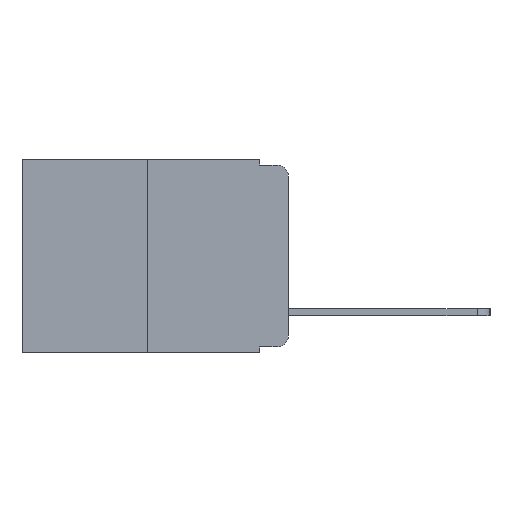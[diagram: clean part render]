
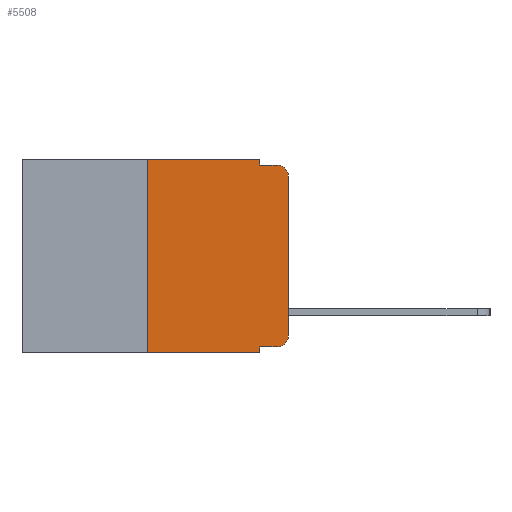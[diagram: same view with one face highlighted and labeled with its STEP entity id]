
A CAD part, left-side view. The second image highlights one B-rep face of the part: STEP entity #5508.
In plain terms, the highlighted planar face has unit normal (-1, 0, 0).
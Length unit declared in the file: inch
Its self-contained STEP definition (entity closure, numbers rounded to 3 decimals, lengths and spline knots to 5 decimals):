
#80 = VECTOR ( 'NONE', #3309, 39.37008 ) ;
#311 = VERTEX_POINT ( 'NONE', #6565 ) ;
#457 = LINE ( 'NONE', #17098, #10699 ) ;
#534 = EDGE_CURVE ( 'NONE', #11161, #9742, #10395, .T. ) ;
#926 = VERTEX_POINT ( 'NONE', #11700 ) ;
#956 = CARTESIAN_POINT ( 'NONE',  ( 0., 0.051, -0.01 ) ) ;
#980 = LINE ( 'NONE', #11636, #11213 ) ;
#1496 = CARTESIAN_POINT ( 'NONE',  ( 0., 0.051, -0.333 ) ) ;
#1633 = ORIENTED_EDGE ( 'NONE', *, *, #11664, .F. ) ;
#1896 = CARTESIAN_POINT ( 'NONE',  ( 0., 0.473, 0. ) ) ;
#2559 = LINE ( 'NONE', #1496, #16178 ) ;
#2613 = ORIENTED_EDGE ( 'NONE', *, *, #13115, .T. ) ;
#3051 = VERTEX_POINT ( 'NONE', #16866 ) ;
#3148 = ORIENTED_EDGE ( 'NONE', *, *, #16303, .F. ) ;
#3309 = DIRECTION ( 'NONE',  ( 0., -1., 0. ) ) ;
#4163 = CARTESIAN_POINT ( 'NONE',  ( 0., 0.02, -0.313 ) ) ;
#4557 = DIRECTION ( 'NONE',  ( 0., 0., -1. ) ) ;
#5054 = CARTESIAN_POINT ( 'NONE',  ( 0., 0.051, 0. ) ) ;
#5508 = ADVANCED_FACE ( 'NONE', ( #12550 ), #9880, .F. ) ;
#5523 = DIRECTION ( 'NONE',  ( 0., 0., -1. ) ) ;
#5671 = CARTESIAN_POINT ( 'NONE',  ( 0., 0.02, -0.03 ) ) ;
#5728 = ORIENTED_EDGE ( 'NONE', *, *, #534, .T. ) ;
#5819 = CARTESIAN_POINT ( 'NONE',  ( 0., 0.25, 0. ) ) ;
#5838 = EDGE_CURVE ( 'NONE', #11592, #9742, #457, .T. ) ;
#6496 = ORIENTED_EDGE ( 'NONE', *, *, #10075, .F. ) ;
#6565 = CARTESIAN_POINT ( 'NONE',  ( 0., 0.051, 0. ) ) ;
#6582 = LINE ( 'NONE', #7953, #13188 ) ;
#6769 = ORIENTED_EDGE ( 'NONE', *, *, #9600, .T. ) ;
#7027 = DIRECTION ( 'NONE',  ( 0., 0., -1. ) ) ;
#7857 = ORIENTED_EDGE ( 'NONE', *, *, #10007, .F. ) ;
#7953 = CARTESIAN_POINT ( 'NONE',  ( 0., 0.051, 0. ) ) ;
#8609 = AXIS2_PLACEMENT_3D ( 'NONE', #1896, #12502, #4557 ) ;
#8787 = VERTEX_POINT ( 'NONE', #11269 ) ;
#8905 = AXIS2_PLACEMENT_3D ( 'NONE', #5671, #14886, #7027 ) ;
#9185 = VERTEX_POINT ( 'NONE', #14641 ) ;
#9314 = DIRECTION ( 'NONE',  ( 0., 0., -1. ) ) ;
#9557 = DIRECTION ( 'NONE',  ( 0., -1., 0. ) ) ;
#9600 = EDGE_CURVE ( 'NONE', #12010, #3051, #980, .T. ) ;
#9742 = VERTEX_POINT ( 'NONE', #10645 ) ;
#9877 = CARTESIAN_POINT ( 'NONE',  ( 0., 0.25, -0.343 ) ) ;
#9880 = PLANE ( 'NONE',  #8609 ) ;
#9894 = CARTESIAN_POINT ( 'NONE',  ( 0., 0.473, 0. ) ) ;
#10007 = EDGE_CURVE ( 'NONE', #12010, #926, #12408, .T. ) ;
#10033 = LINE ( 'NONE', #14863, #13107 ) ;
#10075 = EDGE_CURVE ( 'NONE', #926, #311, #11192, .T. ) ;
#10395 = CIRCLE ( 'NONE', #8905, 0.02 ) ;
#10645 = CARTESIAN_POINT ( 'NONE',  ( 0., 0.02, -0.01 ) ) ;
#10699 = VECTOR ( 'NONE', #15784, 39.37008 ) ;
#11136 = ORIENTED_EDGE ( 'NONE', *, *, #16939, .T. ) ;
#11161 = VERTEX_POINT ( 'NONE', #12073 ) ;
#11192 = LINE ( 'NONE', #9894, #80 ) ;
#11213 = VECTOR ( 'NONE', #12895, 39.37008 ) ;
#11242 = EDGE_CURVE ( 'NONE', #15263, #9185, #2559, .T. ) ;
#11269 = CARTESIAN_POINT ( 'NONE',  ( 0., 0., -0.313 ) ) ;
#11592 = VERTEX_POINT ( 'NONE', #956 ) ;
#11636 = CARTESIAN_POINT ( 'NONE',  ( 0., 0.473, -0.343 ) ) ;
#11664 = EDGE_CURVE ( 'NONE', #15263, #3051, #16581, .T. ) ;
#11700 = CARTESIAN_POINT ( 'NONE',  ( 0., 0.25, 0. ) ) ;
#12010 = VERTEX_POINT ( 'NONE', #9877 ) ;
#12051 = ORIENTED_EDGE ( 'NONE', *, *, #11242, .T. ) ;
#12073 = CARTESIAN_POINT ( 'NONE',  ( 0., 0., -0.03 ) ) ;
#12095 = CARTESIAN_POINT ( 'NONE',  ( 0., 0.051, -0.333 ) ) ;
#12408 = LINE ( 'NONE', #5819, #15046 ) ;
#12502 = DIRECTION ( 'NONE',  ( 1., 0., 0. ) ) ;
#12540 = ORIENTED_EDGE ( 'NONE', *, *, #5838, .F. ) ;
#12550 = FACE_OUTER_BOUND ( 'NONE', #16741, .T. ) ;
#12895 = DIRECTION ( 'NONE',  ( 0., -1., 0. ) ) ;
#13107 = VECTOR ( 'NONE', #14921, 39.37008 ) ;
#13115 = EDGE_CURVE ( 'NONE', #9185, #8787, #17134, .T. ) ;
#13133 = VECTOR ( 'NONE', #16894, 39.37008 ) ;
#13188 = VECTOR ( 'NONE', #9314, 39.37008 ) ;
#13431 = DIRECTION ( 'NONE',  ( -1., 0., 0. ) ) ;
#13726 = DIRECTION ( 'NONE',  ( 0., 0., 1. ) ) ;
#14641 = CARTESIAN_POINT ( 'NONE',  ( 0., 0.02, -0.333 ) ) ;
#14863 = CARTESIAN_POINT ( 'NONE',  ( 0., 0., 0. ) ) ;
#14886 = DIRECTION ( 'NONE',  ( -1., 0., 0. ) ) ;
#14921 = DIRECTION ( 'NONE',  ( 0., 0., 1. ) ) ;
#15046 = VECTOR ( 'NONE', #13726, 39.37008 ) ;
#15263 = VERTEX_POINT ( 'NONE', #12095 ) ;
#15784 = DIRECTION ( 'NONE',  ( 0., -1., 0. ) ) ;
#16142 = AXIS2_PLACEMENT_3D ( 'NONE', #4163, #13431, #5523 ) ;
#16178 = VECTOR ( 'NONE', #9557, 39.37008 ) ;
#16303 = EDGE_CURVE ( 'NONE', #311, #11592, #6582, .T. ) ;
#16581 = LINE ( 'NONE', #5054, #13133 ) ;
#16741 = EDGE_LOOP ( 'NONE', ( #11136, #5728, #12540, #3148, #6496, #7857, #6769, #1633, #12051, #2613 ) ) ;
#16866 = CARTESIAN_POINT ( 'NONE',  ( 0., 0.051, -0.343 ) ) ;
#16894 = DIRECTION ( 'NONE',  ( 0., 0., -1. ) ) ;
#16939 = EDGE_CURVE ( 'NONE', #8787, #11161, #10033, .T. ) ;
#17098 = CARTESIAN_POINT ( 'NONE',  ( 0., 0.051, -0.01 ) ) ;
#17134 = CIRCLE ( 'NONE', #16142, 0.02 ) ;
